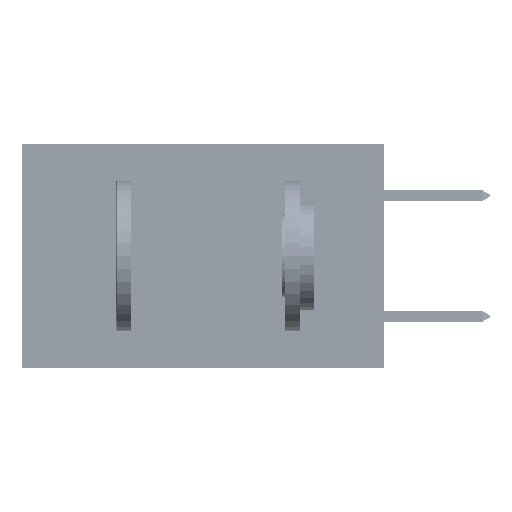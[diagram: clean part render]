
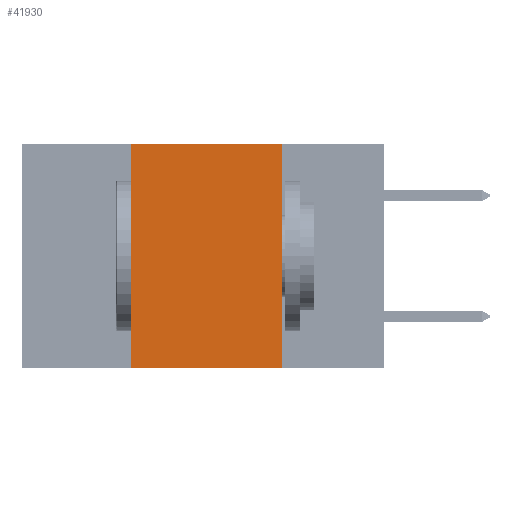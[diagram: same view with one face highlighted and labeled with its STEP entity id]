
A CAD part, left-side view. The second image highlights one B-rep face of the part: STEP entity #41930.
In plain terms, the highlighted planar face has unit normal (-1, 0, 0).
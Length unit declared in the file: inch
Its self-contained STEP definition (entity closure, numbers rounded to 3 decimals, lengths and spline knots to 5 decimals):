
#488 = CARTESIAN_POINT ( 'NONE',  ( 0., 0.17, 0. ) ) ;
#1377 = AXIS2_PLACEMENT_3D ( 'NONE', #21683, #26039, #6344 ) ;
#3664 = CARTESIAN_POINT ( 'NONE',  ( 0., 0.42, -0.37 ) ) ;
#3719 = CARTESIAN_POINT ( 'NONE',  ( 0., 0.17, -0.37 ) ) ;
#4145 = VECTOR ( 'NONE', #21517, 39.37008 ) ;
#6278 = VECTOR ( 'NONE', #39743, 39.37008 ) ;
#6344 = DIRECTION ( 'NONE',  ( 0., 0., -1. ) ) ;
#6703 = LINE ( 'NONE', #17262, #4145 ) ;
#6927 = EDGE_CURVE ( 'NONE', #28440, #11982, #30356, .T. ) ;
#8824 = LINE ( 'NONE', #488, #13206 ) ;
#10030 = PLANE ( 'NONE',  #1377 ) ;
#10658 = LINE ( 'NONE', #39405, #6278 ) ;
#11982 = VERTEX_POINT ( 'NONE', #40057 ) ;
#13206 = VECTOR ( 'NONE', #44252, 39.37008 ) ;
#14658 = VECTOR ( 'NONE', #27404, 39.37008 ) ;
#17150 = ORIENTED_EDGE ( 'NONE', *, *, #39855, .F. ) ;
#17262 = CARTESIAN_POINT ( 'NONE',  ( 0., 0.6, 0. ) ) ;
#18654 = ORIENTED_EDGE ( 'NONE', *, *, #41711, .F. ) ;
#21517 = DIRECTION ( 'NONE',  ( 0., -1., 0. ) ) ;
#21683 = CARTESIAN_POINT ( 'NONE',  ( 0., 0.6, 0. ) ) ;
#26039 = DIRECTION ( 'NONE',  ( 1., 0., 0. ) ) ;
#27404 = DIRECTION ( 'NONE',  ( 0., 0., 1. ) ) ;
#28440 = VERTEX_POINT ( 'NONE', #3664 ) ;
#30356 = LINE ( 'NONE', #47756, #14658 ) ;
#31102 = EDGE_LOOP ( 'NONE', ( #17150, #18654, #34409, #43986 ) ) ;
#34409 = ORIENTED_EDGE ( 'NONE', *, *, #6927, .F. ) ;
#38540 = VERTEX_POINT ( 'NONE', #51102 ) ;
#39405 = CARTESIAN_POINT ( 'NONE',  ( 0., 0.6, -0.37 ) ) ;
#39743 = DIRECTION ( 'NONE',  ( 0., -1., 0. ) ) ;
#39855 = EDGE_CURVE ( 'NONE', #38540, #50337, #8824, .T. ) ;
#40057 = CARTESIAN_POINT ( 'NONE',  ( 0., 0.42, 0. ) ) ;
#41711 = EDGE_CURVE ( 'NONE', #11982, #38540, #6703, .T. ) ;
#41930 = ADVANCED_FACE ( 'NONE', ( #46255 ), #10030, .F. ) ;
#43986 = ORIENTED_EDGE ( 'NONE', *, *, #50435, .T. ) ;
#44252 = DIRECTION ( 'NONE',  ( 0., 0., -1. ) ) ;
#46255 = FACE_OUTER_BOUND ( 'NONE', #31102, .T. ) ;
#47756 = CARTESIAN_POINT ( 'NONE',  ( 0., 0.42, 0. ) ) ;
#50337 = VERTEX_POINT ( 'NONE', #3719 ) ;
#50435 = EDGE_CURVE ( 'NONE', #28440, #50337, #10658, .T. ) ;
#51102 = CARTESIAN_POINT ( 'NONE',  ( 0., 0.17, 0. ) ) ;
